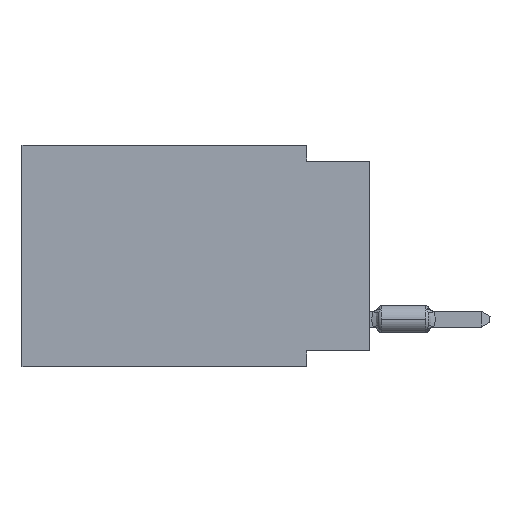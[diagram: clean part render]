
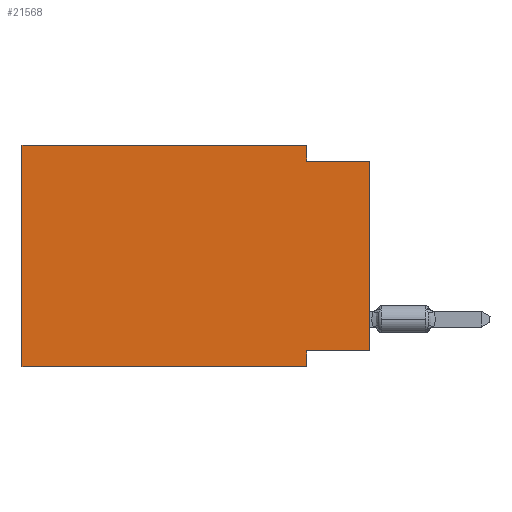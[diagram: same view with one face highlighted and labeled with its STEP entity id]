
A CAD part, left-side view. The second image highlights one B-rep face of the part: STEP entity #21568.
In plain terms, the highlighted planar face has unit normal (-1, 0, 0).
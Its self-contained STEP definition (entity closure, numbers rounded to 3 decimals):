
#104 = VECTOR ( 'NONE', #32787, 1000. ) ;
#530 = LINE ( 'NONE', #28724, #38233 ) ;
#889 = ORIENTED_EDGE ( 'NONE', *, *, #10330, .T. ) ;
#1696 = VERTEX_POINT ( 'NONE', #9277 ) ;
#2004 = LINE ( 'NONE', #60847, #19910 ) ;
#3060 = EDGE_CURVE ( 'NONE', #22036, #12375, #23785, .T. ) ;
#7621 = ORIENTED_EDGE ( 'NONE', *, *, #12190, .F. ) ;
#8440 = CARTESIAN_POINT ( 'NONE',  ( 0., 2.54, -8.89 ) ) ;
#9209 = DIRECTION ( 'NONE',  ( 0., 0., 1. ) ) ;
#9277 = CARTESIAN_POINT ( 'NONE',  ( 0., 2.54, -0.635 ) ) ;
#9307 = EDGE_CURVE ( 'NONE', #1696, #10819, #9344, .T. ) ;
#9344 = LINE ( 'NONE', #34303, #59453 ) ;
#9430 = VECTOR ( 'NONE', #9209, 1000. ) ;
#10014 = AXIS2_PLACEMENT_3D ( 'NONE', #56387, #51284, #32386 ) ;
#10330 = EDGE_CURVE ( 'NONE', #45517, #10819, #53040, .T. ) ;
#10712 = EDGE_LOOP ( 'NONE', ( #889, #63284, #13161, #37078, #7621, #32789, #54779, #16769 ) ) ;
#10819 = VERTEX_POINT ( 'NONE', #41109 ) ;
#12190 = EDGE_CURVE ( 'NONE', #61338, #27000, #530, .T. ) ;
#12375 = VERTEX_POINT ( 'NONE', #61920 ) ;
#13161 = ORIENTED_EDGE ( 'NONE', *, *, #46003, .F. ) ;
#16769 = ORIENTED_EDGE ( 'NONE', *, *, #51612, .F. ) ;
#19739 = CARTESIAN_POINT ( 'NONE',  ( 0., 2.54, 0. ) ) ;
#19910 = VECTOR ( 'NONE', #51571, 1000. ) ;
#21568 = ADVANCED_FACE ( 'NONE', ( #35940 ), #41381, .F. ) ;
#22036 = VERTEX_POINT ( 'NONE', #28474 ) ;
#23785 = LINE ( 'NONE', #8440, #33492 ) ;
#27000 = VERTEX_POINT ( 'NONE', #31449 ) ;
#28474 = CARTESIAN_POINT ( 'NONE',  ( 0., 2.54, -8.255 ) ) ;
#28724 = CARTESIAN_POINT ( 'NONE',  ( 0., 13.97, 0. ) ) ;
#29037 = CARTESIAN_POINT ( 'NONE',  ( 0., 0., 0. ) ) ;
#31449 = CARTESIAN_POINT ( 'NONE',  ( 0., 13.97, 0. ) ) ;
#32386 = DIRECTION ( 'NONE',  ( 0., 0., -1. ) ) ;
#32787 = DIRECTION ( 'NONE',  ( 0., -1., 0. ) ) ;
#32789 = ORIENTED_EDGE ( 'NONE', *, *, #43786, .T. ) ;
#33422 = LINE ( 'NONE', #58036, #104 ) ;
#33492 = VECTOR ( 'NONE', #48738, 1000. ) ;
#33662 = LINE ( 'NONE', #48701, #39726 ) ;
#34303 = CARTESIAN_POINT ( 'NONE',  ( 0., 0., -0.635 ) ) ;
#34781 = DIRECTION ( 'NONE',  ( 0., 0., 1. ) ) ;
#35003 = CARTESIAN_POINT ( 'NONE',  ( 0., 0., -8.255 ) ) ;
#35341 = CARTESIAN_POINT ( 'NONE',  ( 0., 13.97, -8.89 ) ) ;
#35940 = FACE_OUTER_BOUND ( 'NONE', #10712, .T. ) ;
#37078 = ORIENTED_EDGE ( 'NONE', *, *, #63057, .F. ) ;
#38233 = VECTOR ( 'NONE', #34781, 1000. ) ;
#39726 = VECTOR ( 'NONE', #62763, 1000. ) ;
#40342 = LINE ( 'NONE', #44827, #52444 ) ;
#41109 = CARTESIAN_POINT ( 'NONE',  ( 0., 0., -0.635 ) ) ;
#41381 = PLANE ( 'NONE',  #10014 ) ;
#43786 = EDGE_CURVE ( 'NONE', #61338, #12375, #2004, .T. ) ;
#44827 = CARTESIAN_POINT ( 'NONE',  ( 0., 0., -8.255 ) ) ;
#45517 = VERTEX_POINT ( 'NONE', #35003 ) ;
#46003 = EDGE_CURVE ( 'NONE', #59548, #1696, #33662, .T. ) ;
#48701 = CARTESIAN_POINT ( 'NONE',  ( 0., 2.54, 0. ) ) ;
#48738 = DIRECTION ( 'NONE',  ( 0., 0., -1. ) ) ;
#51284 = DIRECTION ( 'NONE',  ( 1., 0., 0. ) ) ;
#51571 = DIRECTION ( 'NONE',  ( 0., -1., 0. ) ) ;
#51612 = EDGE_CURVE ( 'NONE', #45517, #22036, #40342, .T. ) ;
#52444 = VECTOR ( 'NONE', #54712, 1000. ) ;
#53040 = LINE ( 'NONE', #29037, #9430 ) ;
#53499 = DIRECTION ( 'NONE',  ( 0., -1., 0. ) ) ;
#54712 = DIRECTION ( 'NONE',  ( 0., 1., 0. ) ) ;
#54779 = ORIENTED_EDGE ( 'NONE', *, *, #3060, .F. ) ;
#56387 = CARTESIAN_POINT ( 'NONE',  ( 0., 13.97, 0. ) ) ;
#58036 = CARTESIAN_POINT ( 'NONE',  ( 0., 13.97, 0. ) ) ;
#59453 = VECTOR ( 'NONE', #53499, 1000. ) ;
#59548 = VERTEX_POINT ( 'NONE', #19739 ) ;
#60847 = CARTESIAN_POINT ( 'NONE',  ( 0., 13.97, -8.89 ) ) ;
#61338 = VERTEX_POINT ( 'NONE', #35341 ) ;
#61920 = CARTESIAN_POINT ( 'NONE',  ( 0., 2.54, -8.89 ) ) ;
#62763 = DIRECTION ( 'NONE',  ( 0., 0., -1. ) ) ;
#63057 = EDGE_CURVE ( 'NONE', #27000, #59548, #33422, .T. ) ;
#63284 = ORIENTED_EDGE ( 'NONE', *, *, #9307, .F. ) ;
